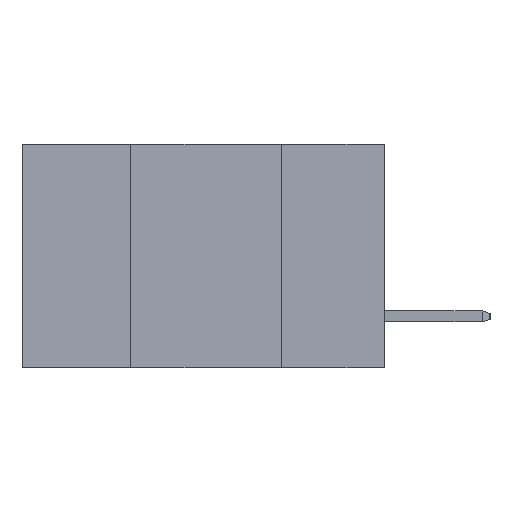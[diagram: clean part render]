
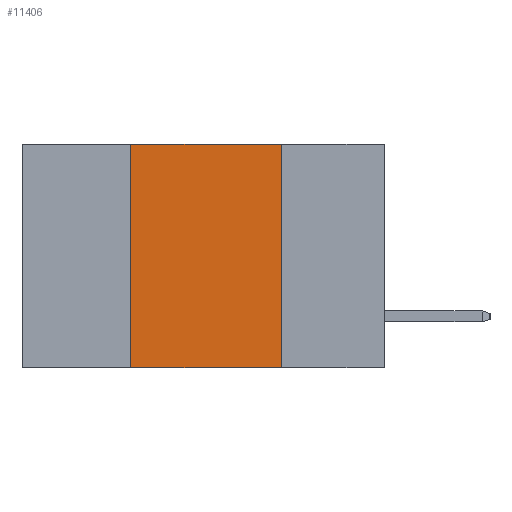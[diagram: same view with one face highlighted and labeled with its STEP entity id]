
A CAD part, left-side view. The second image highlights one B-rep face of the part: STEP entity #11406.
In plain terms, the highlighted planar face has unit normal (-1, 0, 0).
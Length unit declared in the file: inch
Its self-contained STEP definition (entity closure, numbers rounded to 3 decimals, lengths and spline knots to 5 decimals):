
#126 = ORIENTED_EDGE ( 'NONE', *, *, #9309, .F. ) ;
#707 = ORIENTED_EDGE ( 'NONE', *, *, #14454, .F. ) ;
#1835 = VERTEX_POINT ( 'NONE', #8169 ) ;
#2044 = VERTEX_POINT ( 'NONE', #11911 ) ;
#3074 = CARTESIAN_POINT ( 'NONE',  ( 0., 0.6, -0.37 ) ) ;
#3723 = LINE ( 'NONE', #14440, #9667 ) ;
#3805 = LINE ( 'NONE', #15090, #10128 ) ;
#4045 = ORIENTED_EDGE ( 'NONE', *, *, #13735, .F. ) ;
#4234 = VERTEX_POINT ( 'NONE', #9331 ) ;
#4603 = FACE_OUTER_BOUND ( 'NONE', #13439, .T. ) ;
#5001 = DIRECTION ( 'NONE',  ( 0., 0., 1. ) ) ;
#5035 = AXIS2_PLACEMENT_3D ( 'NONE', #13250, #14414, #7357 ) ;
#5069 = LINE ( 'NONE', #3074, #7483 ) ;
#6153 = CARTESIAN_POINT ( 'NONE',  ( 0., 0.42, -0.37 ) ) ;
#6903 = VERTEX_POINT ( 'NONE', #6153 ) ;
#7357 = DIRECTION ( 'NONE',  ( 0., 0., -1. ) ) ;
#7483 = VECTOR ( 'NONE', #12572, 39.37008 ) ;
#8041 = DIRECTION ( 'NONE',  ( 0., -1., 0. ) ) ;
#8169 = CARTESIAN_POINT ( 'NONE',  ( 0., 0.17, 0. ) ) ;
#9309 = EDGE_CURVE ( 'NONE', #1835, #4234, #3723, .T. ) ;
#9331 = CARTESIAN_POINT ( 'NONE',  ( 0., 0.17, -0.37 ) ) ;
#9667 = VECTOR ( 'NONE', #14495, 39.37008 ) ;
#10128 = VECTOR ( 'NONE', #8041, 39.37008 ) ;
#10922 = CARTESIAN_POINT ( 'NONE',  ( 0., 0.42, -0.37 ) ) ;
#11206 = VECTOR ( 'NONE', #5001, 39.37008 ) ;
#11406 = ADVANCED_FACE ( 'NONE', ( #4603 ), #12083, .F. ) ;
#11911 = CARTESIAN_POINT ( 'NONE',  ( 0., 0.42, 0. ) ) ;
#12083 = PLANE ( 'NONE',  #5035 ) ;
#12572 = DIRECTION ( 'NONE',  ( 0., -1., 0. ) ) ;
#13250 = CARTESIAN_POINT ( 'NONE',  ( 0., 0.6, 0. ) ) ;
#13439 = EDGE_LOOP ( 'NONE', ( #126, #4045, #707, #13855 ) ) ;
#13735 = EDGE_CURVE ( 'NONE', #2044, #1835, #3805, .T. ) ;
#13855 = ORIENTED_EDGE ( 'NONE', *, *, #14713, .T. ) ;
#14414 = DIRECTION ( 'NONE',  ( 1., 0., 0. ) ) ;
#14440 = CARTESIAN_POINT ( 'NONE',  ( 0., 0.17, -0.37 ) ) ;
#14454 = EDGE_CURVE ( 'NONE', #6903, #2044, #14679, .T. ) ;
#14495 = DIRECTION ( 'NONE',  ( 0., 0., -1. ) ) ;
#14679 = LINE ( 'NONE', #10922, #11206 ) ;
#14713 = EDGE_CURVE ( 'NONE', #6903, #4234, #5069, .T. ) ;
#15090 = CARTESIAN_POINT ( 'NONE',  ( 0., 0.6, 0. ) ) ;
